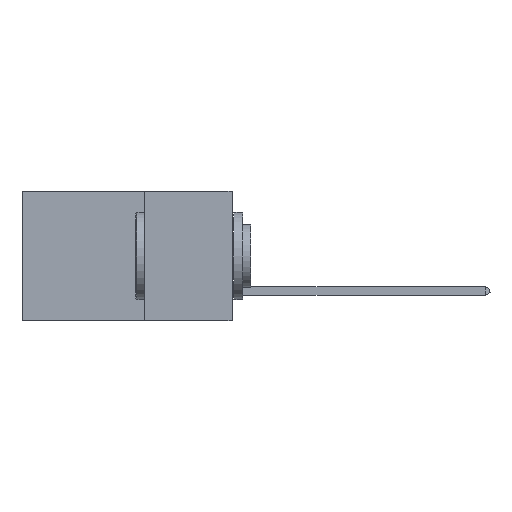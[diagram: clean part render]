
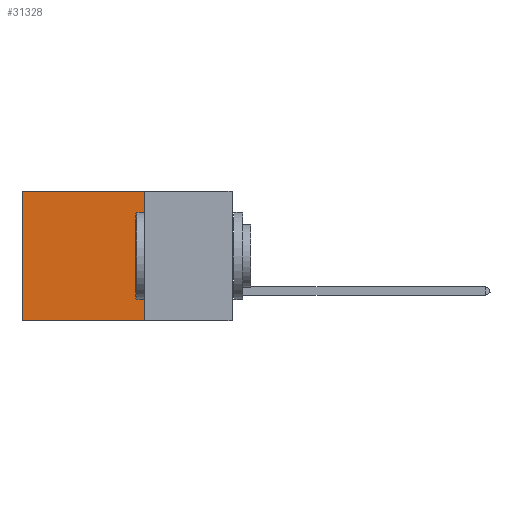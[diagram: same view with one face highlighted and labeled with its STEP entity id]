
A CAD part, left-side view. The second image highlights one B-rep face of the part: STEP entity #31328.
In plain terms, the highlighted planar face has unit normal (-1, 0, 0).
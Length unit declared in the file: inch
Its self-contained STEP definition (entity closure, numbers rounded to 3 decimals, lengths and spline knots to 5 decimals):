
#708 = LINE ( 'NONE', #18476, #32080 ) ;
#836 = CARTESIAN_POINT ( 'NONE',  ( 0.2875, 0.25, -0.37 ) ) ;
#3295 = CARTESIAN_POINT ( 'NONE',  ( 0.2875, 0.6, -0.37 ) ) ;
#3527 = EDGE_CURVE ( 'NONE', #39902, #21574, #40998, .T. ) ;
#7757 = VECTOR ( 'NONE', #20392, 39.37008 ) ;
#8716 = CARTESIAN_POINT ( 'NONE',  ( 0.2875, 0.25, -0.37 ) ) ;
#10438 = ORIENTED_EDGE ( 'NONE', *, *, #38374, .T. ) ;
#14615 = VERTEX_POINT ( 'NONE', #3295 ) ;
#17255 = VECTOR ( 'NONE', #28662, 39.37008 ) ;
#17839 = LINE ( 'NONE', #42949, #7757 ) ;
#18476 = CARTESIAN_POINT ( 'NONE',  ( 0.2875, 0.6, 0. ) ) ;
#20392 = DIRECTION ( 'NONE',  ( 0., 1., 0. ) ) ;
#20719 = CARTESIAN_POINT ( 'NONE',  ( 0.2875, 0.25, 0. ) ) ;
#21574 = VERTEX_POINT ( 'NONE', #836 ) ;
#21743 = DIRECTION ( 'NONE',  ( 1., 0., 0. ) ) ;
#25012 = DIRECTION ( 'NONE',  ( 0., 0., -1. ) ) ;
#25523 = CARTESIAN_POINT ( 'NONE',  ( 0.2875, 0.25, 0. ) ) ;
#26468 = EDGE_CURVE ( 'NONE', #21574, #14615, #41470, .T. ) ;
#27504 = ORIENTED_EDGE ( 'NONE', *, *, #36543, .T. ) ;
#27748 = DIRECTION ( 'NONE',  ( 0., 1., 0. ) ) ;
#27818 = ORIENTED_EDGE ( 'NONE', *, *, #3527, .F. ) ;
#28662 = DIRECTION ( 'NONE',  ( 0., 0., -1. ) ) ;
#29523 = AXIS2_PLACEMENT_3D ( 'NONE', #25523, #21743, #25012 ) ;
#31328 = ADVANCED_FACE ( 'NONE', ( #48548 ), #32991, .F. ) ;
#31554 = CARTESIAN_POINT ( 'NONE',  ( 0.2875, 0.25, 0. ) ) ;
#32080 = VECTOR ( 'NONE', #40839, 39.37008 ) ;
#32504 = CARTESIAN_POINT ( 'NONE',  ( 0.2875, 0.6, 0. ) ) ;
#32991 = PLANE ( 'NONE',  #29523 ) ;
#33640 = EDGE_LOOP ( 'NONE', ( #10438, #36158, #27818, #27504 ) ) ;
#34367 = VECTOR ( 'NONE', #27748, 39.37008 ) ;
#35041 = VERTEX_POINT ( 'NONE', #32504 ) ;
#36158 = ORIENTED_EDGE ( 'NONE', *, *, #26468, .F. ) ;
#36543 = EDGE_CURVE ( 'NONE', #39902, #35041, #17839, .T. ) ;
#38374 = EDGE_CURVE ( 'NONE', #35041, #14615, #708, .T. ) ;
#39902 = VERTEX_POINT ( 'NONE', #31554 ) ;
#40839 = DIRECTION ( 'NONE',  ( 0., 0., -1. ) ) ;
#40998 = LINE ( 'NONE', #20719, #17255 ) ;
#41470 = LINE ( 'NONE', #8716, #34367 ) ;
#42949 = CARTESIAN_POINT ( 'NONE',  ( 0.2875, 0.25, 0. ) ) ;
#48548 = FACE_OUTER_BOUND ( 'NONE', #33640, .T. ) ;
